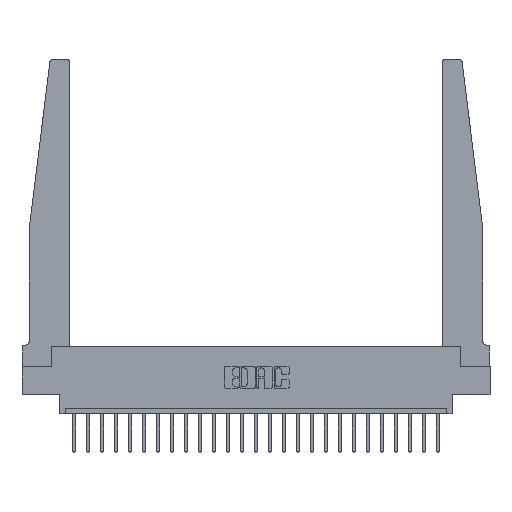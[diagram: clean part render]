
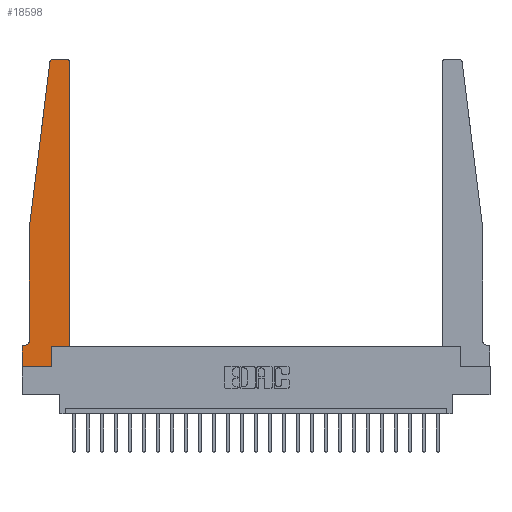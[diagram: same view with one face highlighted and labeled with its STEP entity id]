
A CAD part, top view. The second image highlights one B-rep face of the part: STEP entity #18598.
In plain terms, the highlighted planar face has unit normal (0, 0, 1).
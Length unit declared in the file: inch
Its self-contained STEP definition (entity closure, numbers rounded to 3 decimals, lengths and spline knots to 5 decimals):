
#61 = DIRECTION ( 'NONE',  ( 1., 0., 0. ) ) ;
#178 = DIRECTION ( 'NONE',  ( 0., 1., 0. ) ) ;
#436 = VECTOR ( 'NONE', #23051, 39.37008 ) ;
#600 = CARTESIAN_POINT ( 'NONE',  ( 0.425, 0.18, 0.37 ) ) ;
#707 = ORIENTED_EDGE ( 'NONE', *, *, #2255, .T. ) ;
#771 = VERTEX_POINT ( 'NONE', #18015 ) ;
#1075 = CARTESIAN_POINT ( 'NONE',  ( 0., 0., 0.37 ) ) ;
#1391 = CARTESIAN_POINT ( 'NONE',  ( 0.015, 0.2375, 0.37 ) ) ;
#1398 = DIRECTION ( 'NONE',  ( 1., 0., 0. ) ) ;
#1462 = ORIENTED_EDGE ( 'NONE', *, *, #17636, .T. ) ;
#1845 = VERTEX_POINT ( 'NONE', #13462 ) ;
#1897 = EDGE_CURVE ( 'NONE', #8840, #23131, #20212, .T. ) ;
#2255 = EDGE_CURVE ( 'NONE', #23131, #12563, #23066, .T. ) ;
#2542 = EDGE_CURVE ( 'NONE', #12563, #19240, #3418, .T. ) ;
#2622 = CARTESIAN_POINT ( 'NONE',  ( 0., 0., 0.37 ) ) ;
#2631 = VECTOR ( 'NONE', #18610, 39.37008 ) ;
#2931 = DIRECTION ( 'NONE',  ( -1., 0., 0. ) ) ;
#3372 = LINE ( 'NONE', #5682, #19151 ) ;
#3418 = LINE ( 'NONE', #12364, #17491 ) ;
#3770 = CARTESIAN_POINT ( 'NONE',  ( 0.065, 1.25, 0.37 ) ) ;
#4098 = VECTOR ( 'NONE', #10957, 39.37008 ) ;
#4160 = CARTESIAN_POINT ( 'NONE',  ( 0.065, 1.25, 0.37 ) ) ;
#4216 = VERTEX_POINT ( 'NONE', #9158 ) ;
#5131 = CARTESIAN_POINT ( 'NONE',  ( 0.395, 2.72, 0.37 ) ) ;
#5226 = AXIS2_PLACEMENT_3D ( 'NONE', #7488, #16423, #61 ) ;
#5311 = VERTEX_POINT ( 'NONE', #18508 ) ;
#5440 = ORIENTED_EDGE ( 'NONE', *, *, #22359, .T. ) ;
#5682 = CARTESIAN_POINT ( 'NONE',  ( 0.2605, 0.18, 0.37 ) ) ;
#5774 = LINE ( 'NONE', #600, #2631 ) ;
#5926 = DIRECTION ( 'NONE',  ( 1., 0., 0. ) ) ;
#6010 = EDGE_CURVE ( 'NONE', #14953, #7172, #9859, .T. ) ;
#6932 = DIRECTION ( 'NONE',  ( -1., 0., 0. ) ) ;
#6967 = AXIS2_PLACEMENT_3D ( 'NONE', #5131, #21617, #10651 ) ;
#7080 = VERTEX_POINT ( 'NONE', #22480 ) ;
#7172 = VERTEX_POINT ( 'NONE', #23251 ) ;
#7488 = CARTESIAN_POINT ( 'NONE',  ( 0., 0.1875, 0.37 ) ) ;
#7820 = EDGE_CURVE ( 'NONE', #7172, #1845, #5774, .T. ) ;
#8759 = ORIENTED_EDGE ( 'NONE', *, *, #14900, .T. ) ;
#8840 = VERTEX_POINT ( 'NONE', #9178 ) ;
#9158 = CARTESIAN_POINT ( 'NONE',  ( 0.395, 2.75, 0.37 ) ) ;
#9178 = CARTESIAN_POINT ( 'NONE',  ( 0.015, 0.1875, 0.37 ) ) ;
#9384 = EDGE_CURVE ( 'NONE', #1845, #4216, #15954, .T. ) ;
#9859 = LINE ( 'NONE', #10470, #436 ) ;
#10120 = CARTESIAN_POINT ( 'NONE',  ( 0.25, 2.75, 0.37 ) ) ;
#10470 = CARTESIAN_POINT ( 'NONE',  ( 0.425, 0.18, 0.37 ) ) ;
#10651 = DIRECTION ( 'NONE',  ( 1., 0., 0. ) ) ;
#10957 = DIRECTION ( 'NONE',  ( -0.122, -0.992, 0. ) ) ;
#11540 = ORIENTED_EDGE ( 'NONE', *, *, #23434, .T. ) ;
#11645 = CARTESIAN_POINT ( 'NONE',  ( 0.27653, 2.75, 0.37 ) ) ;
#11809 = DIRECTION ( 'NONE',  ( -1., 0., 0. ) ) ;
#12358 = DIRECTION ( 'NONE',  ( 0., 0., -1. ) ) ;
#12364 = CARTESIAN_POINT ( 'NONE',  ( 0., 0., 0.37 ) ) ;
#12532 = CARTESIAN_POINT ( 'NONE',  ( 0., 0.1875, 0.37 ) ) ;
#12563 = VERTEX_POINT ( 'NONE', #2622 ) ;
#13097 = LINE ( 'NONE', #10120, #18561 ) ;
#13462 = CARTESIAN_POINT ( 'NONE',  ( 0.425, 2.72, 0.37 ) ) ;
#13603 = CARTESIAN_POINT ( 'NONE',  ( 0.065, 0.1875, 0.37 ) ) ;
#13916 = DIRECTION ( 'NONE',  ( 0., -1., 0. ) ) ;
#14273 = AXIS2_PLACEMENT_3D ( 'NONE', #1391, #12358, #6932 ) ;
#14616 = ORIENTED_EDGE ( 'NONE', *, *, #9384, .T. ) ;
#14900 = EDGE_CURVE ( 'NONE', #19240, #14953, #3372, .T. ) ;
#14953 = VERTEX_POINT ( 'NONE', #19131 ) ;
#15147 = FACE_OUTER_BOUND ( 'NONE', #20593, .T. ) ;
#15533 = ORIENTED_EDGE ( 'NONE', *, *, #23379, .T. ) ;
#15781 = CARTESIAN_POINT ( 'NONE',  ( 0.2605, 0., 0.37 ) ) ;
#15954 = CIRCLE ( 'NONE', #6967, 0.03 ) ;
#16423 = DIRECTION ( 'NONE',  ( 0., 0., 1. ) ) ;
#16622 = PLANE ( 'NONE',  #5226 ) ;
#16919 = DIRECTION ( 'NONE',  ( 0., 0., 1. ) ) ;
#16947 = ORIENTED_EDGE ( 'NONE', *, *, #1897, .T. ) ;
#17462 = ORIENTED_EDGE ( 'NONE', *, *, #7820, .T. ) ;
#17491 = VECTOR ( 'NONE', #1398, 39.37008 ) ;
#17636 = EDGE_CURVE ( 'NONE', #7080, #771, #22620, .T. ) ;
#18015 = CARTESIAN_POINT ( 'NONE',  ( 0.065, 0.2375, 0.37 ) ) ;
#18233 = VECTOR ( 'NONE', #13916, 39.37008 ) ;
#18508 = CARTESIAN_POINT ( 'NONE',  ( 0.24675, 2.72367, 0.37 ) ) ;
#18516 = VECTOR ( 'NONE', #2931, 39.37008 ) ;
#18561 = VECTOR ( 'NONE', #11809, 39.37008 ) ;
#18598 = ADVANCED_FACE ( 'NONE', ( #15147 ), #16622, .T. ) ;
#18610 = DIRECTION ( 'NONE',  ( 0., 1., 0. ) ) ;
#18851 = ORIENTED_EDGE ( 'NONE', *, *, #2542, .T. ) ;
#19131 = CARTESIAN_POINT ( 'NONE',  ( 0.2605, 0.18, 0.37 ) ) ;
#19151 = VECTOR ( 'NONE', #178, 39.37008 ) ;
#19211 = CIRCLE ( 'NONE', #19834, 0.03 ) ;
#19240 = VERTEX_POINT ( 'NONE', #15781 ) ;
#19352 = ORIENTED_EDGE ( 'NONE', *, *, #22103, .T. ) ;
#19834 = AXIS2_PLACEMENT_3D ( 'NONE', #20551, #16919, #5926 ) ;
#19972 = CIRCLE ( 'NONE', #14273, 0.05 ) ;
#20212 = LINE ( 'NONE', #13603, #18516 ) ;
#20551 = CARTESIAN_POINT ( 'NONE',  ( 0.27653, 2.72, 0.37 ) ) ;
#20593 = EDGE_LOOP ( 'NONE', ( #15533, #5440, #19352, #1462, #11540, #16947, #707, #18851, #8759, #22842, #17462, #14616 ) ) ;
#20700 = LINE ( 'NONE', #3770, #4098 ) ;
#21129 = VERTEX_POINT ( 'NONE', #11645 ) ;
#21617 = DIRECTION ( 'NONE',  ( 0., 0., 1. ) ) ;
#22103 = EDGE_CURVE ( 'NONE', #5311, #7080, #20700, .T. ) ;
#22359 = EDGE_CURVE ( 'NONE', #21129, #5311, #19211, .T. ) ;
#22413 = DIRECTION ( 'NONE',  ( 0., -1., 0. ) ) ;
#22480 = CARTESIAN_POINT ( 'NONE',  ( 0.065, 1.25, 0.37 ) ) ;
#22620 = LINE ( 'NONE', #4160, #22891 ) ;
#22842 = ORIENTED_EDGE ( 'NONE', *, *, #6010, .T. ) ;
#22891 = VECTOR ( 'NONE', #22413, 39.37008 ) ;
#23051 = DIRECTION ( 'NONE',  ( 1., 0., 0. ) ) ;
#23066 = LINE ( 'NONE', #1075, #18233 ) ;
#23131 = VERTEX_POINT ( 'NONE', #12532 ) ;
#23251 = CARTESIAN_POINT ( 'NONE',  ( 0.425, 0.18, 0.37 ) ) ;
#23379 = EDGE_CURVE ( 'NONE', #4216, #21129, #13097, .T. ) ;
#23434 = EDGE_CURVE ( 'NONE', #771, #8840, #19972, .T. ) ;
